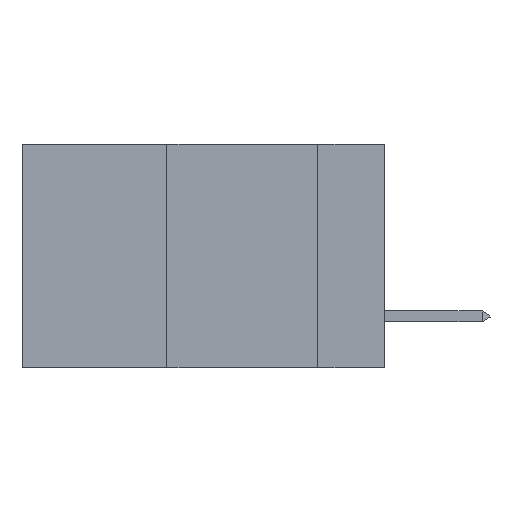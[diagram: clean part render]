
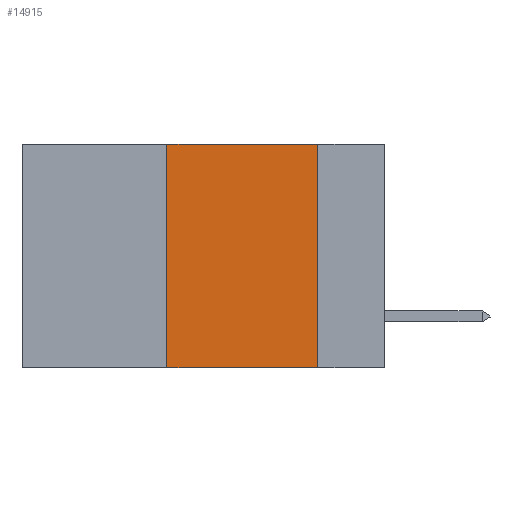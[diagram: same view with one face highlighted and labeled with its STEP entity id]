
A CAD part, left-side view. The second image highlights one B-rep face of the part: STEP entity #14915.
In plain terms, the highlighted planar face has unit normal (-1, 0, 0).
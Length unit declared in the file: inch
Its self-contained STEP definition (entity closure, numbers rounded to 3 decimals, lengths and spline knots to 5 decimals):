
#1741 = ORIENTED_EDGE ( 'NONE', *, *, #17619, .F. ) ;
#2613 = EDGE_CURVE ( 'NONE', #14491, #9267, #8862, .T. ) ;
#2745 = LINE ( 'NONE', #20521, #6447 ) ;
#4095 = DIRECTION ( 'NONE',  ( 0., -1., 0. ) ) ;
#4733 = DIRECTION ( 'NONE',  ( 0., 0., -1. ) ) ;
#4838 = EDGE_CURVE ( 'NONE', #10348, #14491, #5028, .T. ) ;
#5028 = LINE ( 'NONE', #7683, #22304 ) ;
#5078 = CARTESIAN_POINT ( 'NONE',  ( 0., 0.11, 0. ) ) ;
#6018 = FACE_OUTER_BOUND ( 'NONE', #9748, .T. ) ;
#6447 = VECTOR ( 'NONE', #7752, 39.37008 ) ;
#7176 = VECTOR ( 'NONE', #21824, 39.37008 ) ;
#7279 = ORIENTED_EDGE ( 'NONE', *, *, #4838, .F. ) ;
#7559 = VERTEX_POINT ( 'NONE', #12234 ) ;
#7683 = CARTESIAN_POINT ( 'NONE',  ( 0., 0.6, 0. ) ) ;
#7752 = DIRECTION ( 'NONE',  ( 0., 0., 1. ) ) ;
#8274 = AXIS2_PLACEMENT_3D ( 'NONE', #14255, #17704, #4733 ) ;
#8862 = LINE ( 'NONE', #15453, #13752 ) ;
#8920 = CARTESIAN_POINT ( 'NONE',  ( 0., 0.6, -0.37 ) ) ;
#9267 = VERTEX_POINT ( 'NONE', #11402 ) ;
#9748 = EDGE_LOOP ( 'NONE', ( #19054, #7279, #1741, #18668 ) ) ;
#9970 = DIRECTION ( 'NONE',  ( 0., 0., -1. ) ) ;
#10348 = VERTEX_POINT ( 'NONE', #13438 ) ;
#11402 = CARTESIAN_POINT ( 'NONE',  ( 0., 0.11, -0.37 ) ) ;
#12234 = CARTESIAN_POINT ( 'NONE',  ( 0., 0.36, -0.37 ) ) ;
#13438 = CARTESIAN_POINT ( 'NONE',  ( 0., 0.36, 0. ) ) ;
#13752 = VECTOR ( 'NONE', #9970, 39.37008 ) ;
#14255 = CARTESIAN_POINT ( 'NONE',  ( 0., 0.6, 0. ) ) ;
#14491 = VERTEX_POINT ( 'NONE', #5078 ) ;
#14915 = ADVANCED_FACE ( 'NONE', ( #6018 ), #23443, .F. ) ;
#15301 = EDGE_CURVE ( 'NONE', #7559, #9267, #20165, .T. ) ;
#15453 = CARTESIAN_POINT ( 'NONE',  ( 0., 0.11, 0. ) ) ;
#17619 = EDGE_CURVE ( 'NONE', #7559, #10348, #2745, .T. ) ;
#17704 = DIRECTION ( 'NONE',  ( 1., 0., 0. ) ) ;
#18668 = ORIENTED_EDGE ( 'NONE', *, *, #15301, .T. ) ;
#19054 = ORIENTED_EDGE ( 'NONE', *, *, #2613, .F. ) ;
#20165 = LINE ( 'NONE', #8920, #7176 ) ;
#20521 = CARTESIAN_POINT ( 'NONE',  ( 0., 0.36, 0. ) ) ;
#21824 = DIRECTION ( 'NONE',  ( 0., -1., 0. ) ) ;
#22304 = VECTOR ( 'NONE', #4095, 39.37008 ) ;
#23443 = PLANE ( 'NONE',  #8274 ) ;
